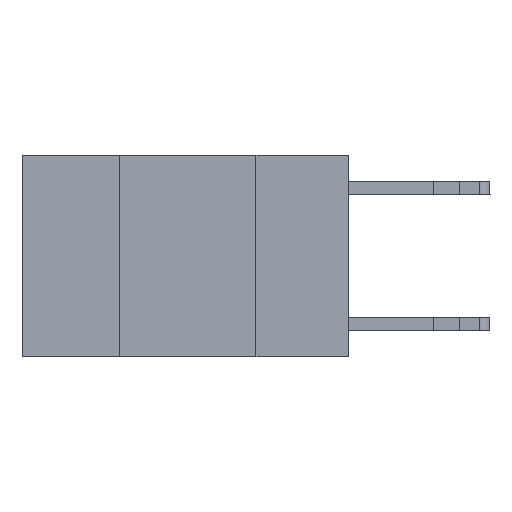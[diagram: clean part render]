
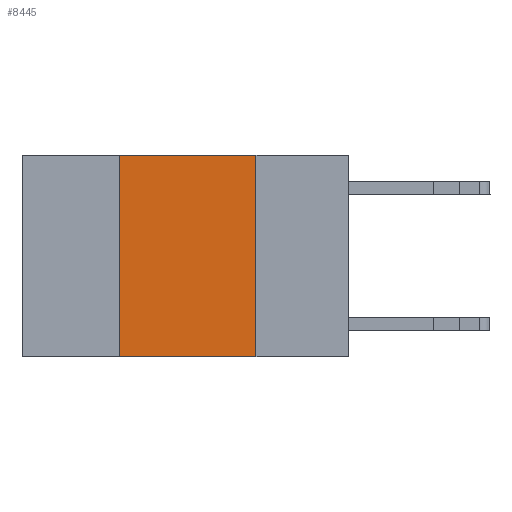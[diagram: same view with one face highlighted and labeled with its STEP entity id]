
A CAD part, left-side view. The second image highlights one B-rep face of the part: STEP entity #8445.
In plain terms, the highlighted planar face has unit normal (-1, 0, 0).
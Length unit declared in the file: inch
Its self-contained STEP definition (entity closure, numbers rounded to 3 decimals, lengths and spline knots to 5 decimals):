
#301 = VECTOR ( 'NONE', #2190, 39.37008 ) ;
#532 = ORIENTED_EDGE ( 'NONE', *, *, #8031, .T. ) ;
#538 = CARTESIAN_POINT ( 'NONE',  ( 0., 0.17, 0. ) ) ;
#893 = EDGE_CURVE ( 'NONE', #2556, #7208, #5427, .T. ) ;
#1021 = EDGE_LOOP ( 'NONE', ( #8402, #3852, #6352, #532 ) ) ;
#1177 = CARTESIAN_POINT ( 'NONE',  ( 0., 0.6, 0. ) ) ;
#1878 = PLANE ( 'NONE',  #5511 ) ;
#2190 = DIRECTION ( 'NONE',  ( 0., -1., 0. ) ) ;
#2318 = EDGE_CURVE ( 'NONE', #9411, #8848, #2927, .T. ) ;
#2345 = VECTOR ( 'NONE', #9337, 39.37008 ) ;
#2556 = VERTEX_POINT ( 'NONE', #7003 ) ;
#2927 = LINE ( 'NONE', #13149, #8037 ) ;
#3218 = LINE ( 'NONE', #1177, #301 ) ;
#3852 = ORIENTED_EDGE ( 'NONE', *, *, #7127, .F. ) ;
#4044 = DIRECTION ( 'NONE',  ( 0., 0., -1. ) ) ;
#4277 = VECTOR ( 'NONE', #10284, 39.37008 ) ;
#5006 = CARTESIAN_POINT ( 'NONE',  ( 0., 0.42, 0. ) ) ;
#5198 = CARTESIAN_POINT ( 'NONE',  ( 0., 0.42, 0. ) ) ;
#5427 = LINE ( 'NONE', #5198, #2345 ) ;
#5511 = AXIS2_PLACEMENT_3D ( 'NONE', #6141, #6074, #4044 ) ;
#6017 = CARTESIAN_POINT ( 'NONE',  ( 0., 0.17, -0.37 ) ) ;
#6074 = DIRECTION ( 'NONE',  ( 1., 0., 0. ) ) ;
#6141 = CARTESIAN_POINT ( 'NONE',  ( 0., 0.6, 0. ) ) ;
#6352 = ORIENTED_EDGE ( 'NONE', *, *, #893, .F. ) ;
#7003 = CARTESIAN_POINT ( 'NONE',  ( 0., 0.42, -0.37 ) ) ;
#7127 = EDGE_CURVE ( 'NONE', #7208, #9411, #3218, .T. ) ;
#7208 = VERTEX_POINT ( 'NONE', #5006 ) ;
#8031 = EDGE_CURVE ( 'NONE', #2556, #8848, #11309, .T. ) ;
#8037 = VECTOR ( 'NONE', #10285, 39.37008 ) ;
#8402 = ORIENTED_EDGE ( 'NONE', *, *, #2318, .F. ) ;
#8445 = ADVANCED_FACE ( 'NONE', ( #11229 ), #1878, .F. ) ;
#8848 = VERTEX_POINT ( 'NONE', #6017 ) ;
#9184 = CARTESIAN_POINT ( 'NONE',  ( 0., 0.6, -0.37 ) ) ;
#9337 = DIRECTION ( 'NONE',  ( 0., 0., 1. ) ) ;
#9411 = VERTEX_POINT ( 'NONE', #538 ) ;
#10284 = DIRECTION ( 'NONE',  ( 0., -1., 0. ) ) ;
#10285 = DIRECTION ( 'NONE',  ( 0., 0., -1. ) ) ;
#11229 = FACE_OUTER_BOUND ( 'NONE', #1021, .T. ) ;
#11309 = LINE ( 'NONE', #9184, #4277 ) ;
#13149 = CARTESIAN_POINT ( 'NONE',  ( 0., 0.17, 0. ) ) ;
